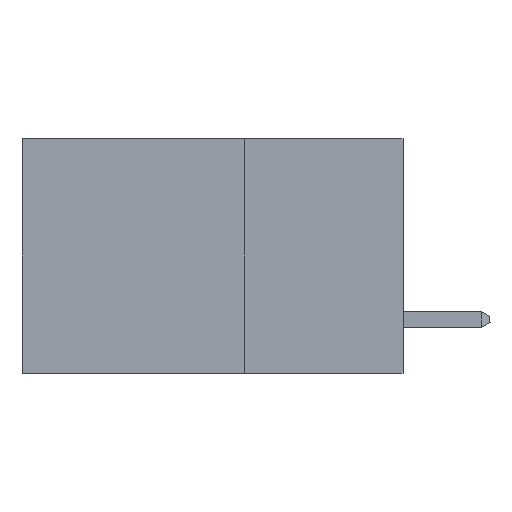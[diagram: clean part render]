
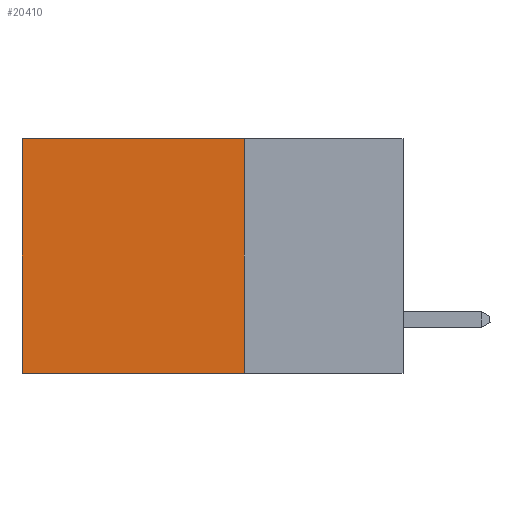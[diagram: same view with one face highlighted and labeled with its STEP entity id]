
A CAD part, left-side view. The second image highlights one B-rep face of the part: STEP entity #20410.
In plain terms, the highlighted planar face has unit normal (-1, 0, 0).
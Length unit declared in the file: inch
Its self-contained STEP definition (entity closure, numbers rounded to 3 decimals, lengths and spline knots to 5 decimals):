
#288 = ORIENTED_EDGE ( 'NONE', *, *, #17964, .T. ) ;
#372 = CARTESIAN_POINT ( 'NONE',  ( 0.2875, 0.25, 0. ) ) ;
#2274 = DIRECTION ( 'NONE',  ( 0., 1., 0. ) ) ;
#2502 = CARTESIAN_POINT ( 'NONE',  ( 0.2875, 0.25, -0.37 ) ) ;
#3402 = PLANE ( 'NONE',  #14012 ) ;
#3755 = DIRECTION ( 'NONE',  ( 1., 0., 0. ) ) ;
#3846 = LINE ( 'NONE', #372, #15239 ) ;
#4372 = LINE ( 'NONE', #2502, #22719 ) ;
#4579 = CARTESIAN_POINT ( 'NONE',  ( 0.2875, 0.25, 0. ) ) ;
#5204 = CARTESIAN_POINT ( 'NONE',  ( 0.2875, 0.25, 0. ) ) ;
#5281 = VERTEX_POINT ( 'NONE', #6051 ) ;
#5577 = DIRECTION ( 'NONE',  ( 0., 0., -1. ) ) ;
#6051 = CARTESIAN_POINT ( 'NONE',  ( 0.2875, 0.6, -0.37 ) ) ;
#6800 = DIRECTION ( 'NONE',  ( 0., 0., -1. ) ) ;
#7942 = DIRECTION ( 'NONE',  ( 0., 1., 0. ) ) ;
#9005 = EDGE_CURVE ( 'NONE', #21713, #5281, #14278, .T. ) ;
#9521 = VECTOR ( 'NONE', #13738, 39.37008 ) ;
#10168 = CARTESIAN_POINT ( 'NONE',  ( 0.2875, 0.25, -0.37 ) ) ;
#12087 = VECTOR ( 'NONE', #6800, 39.37008 ) ;
#13161 = LINE ( 'NONE', #13787, #12087 ) ;
#13738 = DIRECTION ( 'NONE',  ( 0., 0., -1. ) ) ;
#13787 = CARTESIAN_POINT ( 'NONE',  ( 0.2875, 0.25, 0. ) ) ;
#14012 = AXIS2_PLACEMENT_3D ( 'NONE', #5204, #3755, #5577 ) ;
#14278 = LINE ( 'NONE', #22051, #9521 ) ;
#15239 = VECTOR ( 'NONE', #7942, 39.37008 ) ;
#16283 = ORIENTED_EDGE ( 'NONE', *, *, #18125, .F. ) ;
#17060 = FACE_OUTER_BOUND ( 'NONE', #21227, .T. ) ;
#17356 = ORIENTED_EDGE ( 'NONE', *, *, #22402, .F. ) ;
#17964 = EDGE_CURVE ( 'NONE', #21776, #21713, #3846, .T. ) ;
#18125 = EDGE_CURVE ( 'NONE', #21537, #5281, #4372, .T. ) ;
#18127 = ORIENTED_EDGE ( 'NONE', *, *, #9005, .T. ) ;
#20410 = ADVANCED_FACE ( 'NONE', ( #17060 ), #3402, .F. ) ;
#21227 = EDGE_LOOP ( 'NONE', ( #18127, #16283, #17356, #288 ) ) ;
#21537 = VERTEX_POINT ( 'NONE', #10168 ) ;
#21713 = VERTEX_POINT ( 'NONE', #22908 ) ;
#21776 = VERTEX_POINT ( 'NONE', #4579 ) ;
#22051 = CARTESIAN_POINT ( 'NONE',  ( 0.2875, 0.6, 0. ) ) ;
#22402 = EDGE_CURVE ( 'NONE', #21776, #21537, #13161, .T. ) ;
#22719 = VECTOR ( 'NONE', #2274, 39.37008 ) ;
#22908 = CARTESIAN_POINT ( 'NONE',  ( 0.2875, 0.6, 0. ) ) ;
